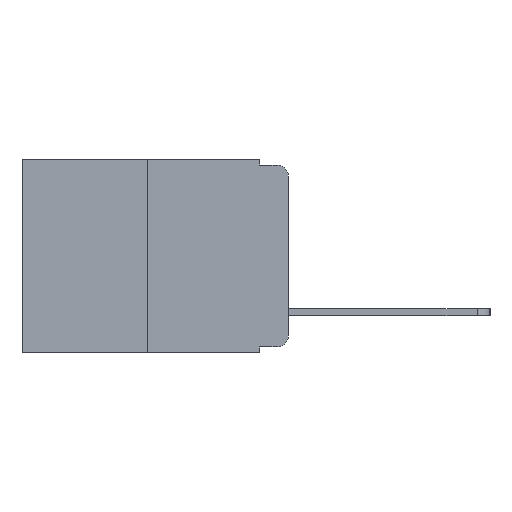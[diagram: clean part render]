
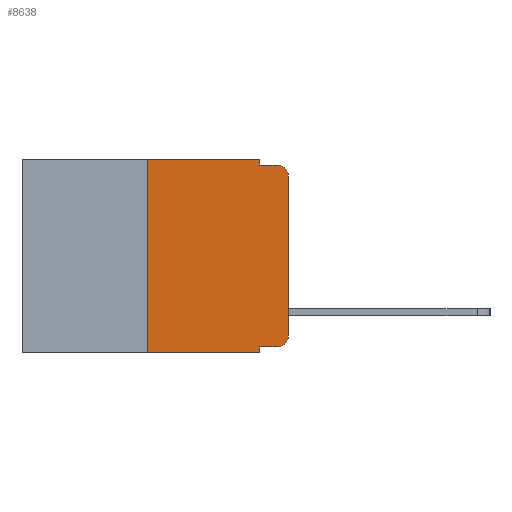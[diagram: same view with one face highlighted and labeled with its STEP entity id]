
A CAD part, left-side view. The second image highlights one B-rep face of the part: STEP entity #8638.
In plain terms, the highlighted planar face has unit normal (-1, 0, 0).
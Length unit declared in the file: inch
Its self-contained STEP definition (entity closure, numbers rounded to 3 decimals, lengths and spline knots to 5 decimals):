
#238 = ORIENTED_EDGE ( 'NONE', *, *, #7026, .T. ) ;
#520 = CARTESIAN_POINT ( 'NONE',  ( 0., 0.02, -0.01 ) ) ;
#692 = VERTEX_POINT ( 'NONE', #14526 ) ;
#790 = AXIS2_PLACEMENT_3D ( 'NONE', #9819, #8954, #10452 ) ;
#845 = CARTESIAN_POINT ( 'NONE',  ( 0., 0.051, -0.343 ) ) ;
#1136 = EDGE_CURVE ( 'NONE', #4900, #7014, #1927, .T. ) ;
#1307 = EDGE_CURVE ( 'NONE', #6296, #9072, #5280, .T. ) ;
#1420 = VERTEX_POINT ( 'NONE', #9366 ) ;
#1461 = VECTOR ( 'NONE', #11084, 39.37008 ) ;
#1786 = VERTEX_POINT ( 'NONE', #845 ) ;
#1927 = LINE ( 'NONE', #8171, #4402 ) ;
#2137 = DIRECTION ( 'NONE',  ( 0., 0., 1. ) ) ;
#2161 = EDGE_CURVE ( 'NONE', #1420, #6296, #7194, .T. ) ;
#2955 = EDGE_CURVE ( 'NONE', #1420, #1786, #13130, .T. ) ;
#3192 = VECTOR ( 'NONE', #13344, 39.37008 ) ;
#3286 = EDGE_LOOP ( 'NONE', ( #238, #3532, #9862, #3923, #10218, #7521, #10550, #4678, #7887, #10880 ) ) ;
#3414 = LINE ( 'NONE', #9518, #6639 ) ;
#3532 = ORIENTED_EDGE ( 'NONE', *, *, #6193, .T. ) ;
#3570 = DIRECTION ( 'NONE',  ( 0., 0., 1. ) ) ;
#3774 = EDGE_CURVE ( 'NONE', #8325, #4900, #13782, .T. ) ;
#3923 = ORIENTED_EDGE ( 'NONE', *, *, #4597, .F. ) ;
#3957 = VERTEX_POINT ( 'NONE', #3966 ) ;
#3966 = CARTESIAN_POINT ( 'NONE',  ( 0., 0.051, -0.01 ) ) ;
#4151 = VERTEX_POINT ( 'NONE', #520 ) ;
#4402 = VECTOR ( 'NONE', #12120, 39.37008 ) ;
#4597 = EDGE_CURVE ( 'NONE', #7014, #3957, #11604, .T. ) ;
#4678 = ORIENTED_EDGE ( 'NONE', *, *, #2955, .F. ) ;
#4755 = DIRECTION ( 'NONE',  ( 1., 0., 0. ) ) ;
#4900 = VERTEX_POINT ( 'NONE', #9797 ) ;
#4984 = CARTESIAN_POINT ( 'NONE',  ( 0., 0.051, 0. ) ) ;
#5280 = CIRCLE ( 'NONE', #7171, 0.02 ) ;
#5340 = EDGE_CURVE ( 'NONE', #3957, #4151, #7539, .T. ) ;
#5543 = VECTOR ( 'NONE', #12682, 39.37008 ) ;
#5758 = DIRECTION ( 'NONE',  ( 0., -1., 0. ) ) ;
#5847 = CARTESIAN_POINT ( 'NONE',  ( 0., 0.473, -0.343 ) ) ;
#5902 = CARTESIAN_POINT ( 'NONE',  ( 0., 0.473, 0. ) ) ;
#6043 = CARTESIAN_POINT ( 'NONE',  ( 0., 0.02, -0.333 ) ) ;
#6193 = EDGE_CURVE ( 'NONE', #692, #4151, #8879, .T. ) ;
#6296 = VERTEX_POINT ( 'NONE', #6043 ) ;
#6639 = VECTOR ( 'NONE', #3570, 39.37008 ) ;
#7014 = VERTEX_POINT ( 'NONE', #7164 ) ;
#7026 = EDGE_CURVE ( 'NONE', #9072, #692, #3414, .T. ) ;
#7164 = CARTESIAN_POINT ( 'NONE',  ( 0., 0.051, 0. ) ) ;
#7171 = AXIS2_PLACEMENT_3D ( 'NONE', #14013, #14075, #14631 ) ;
#7194 = LINE ( 'NONE', #11792, #12797 ) ;
#7521 = ORIENTED_EDGE ( 'NONE', *, *, #3774, .F. ) ;
#7539 = LINE ( 'NONE', #13043, #1461 ) ;
#7887 = ORIENTED_EDGE ( 'NONE', *, *, #2161, .T. ) ;
#7933 = VECTOR ( 'NONE', #2137, 39.37008 ) ;
#8015 = FACE_OUTER_BOUND ( 'NONE', #3286, .T. ) ;
#8171 = CARTESIAN_POINT ( 'NONE',  ( 0., 0.473, 0. ) ) ;
#8325 = VERTEX_POINT ( 'NONE', #13309 ) ;
#8364 = DIRECTION ( 'NONE',  ( 0., 0., -1. ) ) ;
#8397 = LINE ( 'NONE', #5847, #5543 ) ;
#8638 = ADVANCED_FACE ( 'NONE', ( #8015 ), #9487, .F. ) ;
#8879 = CIRCLE ( 'NONE', #790, 0.02 ) ;
#8954 = DIRECTION ( 'NONE',  ( -1., 0., 0. ) ) ;
#9072 = VERTEX_POINT ( 'NONE', #13862 ) ;
#9366 = CARTESIAN_POINT ( 'NONE',  ( 0., 0.051, -0.333 ) ) ;
#9487 = PLANE ( 'NONE',  #10616 ) ;
#9518 = CARTESIAN_POINT ( 'NONE',  ( 0., 0., 0. ) ) ;
#9797 = CARTESIAN_POINT ( 'NONE',  ( 0., 0.25, 0. ) ) ;
#9819 = CARTESIAN_POINT ( 'NONE',  ( 0., 0.02, -0.03 ) ) ;
#9862 = ORIENTED_EDGE ( 'NONE', *, *, #5340, .F. ) ;
#10218 = ORIENTED_EDGE ( 'NONE', *, *, #1136, .F. ) ;
#10452 = DIRECTION ( 'NONE',  ( 0., 0., -1. ) ) ;
#10550 = ORIENTED_EDGE ( 'NONE', *, *, #14178, .T. ) ;
#10616 = AXIS2_PLACEMENT_3D ( 'NONE', #5902, #4755, #12763 ) ;
#10880 = ORIENTED_EDGE ( 'NONE', *, *, #1307, .T. ) ;
#10910 = CARTESIAN_POINT ( 'NONE',  ( 0., 0.25, 0. ) ) ;
#11084 = DIRECTION ( 'NONE',  ( 0., -1., 0. ) ) ;
#11604 = LINE ( 'NONE', #13112, #14104 ) ;
#11792 = CARTESIAN_POINT ( 'NONE',  ( 0., 0.051, -0.333 ) ) ;
#12120 = DIRECTION ( 'NONE',  ( 0., -1., 0. ) ) ;
#12682 = DIRECTION ( 'NONE',  ( 0., -1., 0. ) ) ;
#12763 = DIRECTION ( 'NONE',  ( 0., 0., -1. ) ) ;
#12797 = VECTOR ( 'NONE', #5758, 39.37008 ) ;
#13043 = CARTESIAN_POINT ( 'NONE',  ( 0., 0.051, -0.01 ) ) ;
#13112 = CARTESIAN_POINT ( 'NONE',  ( 0., 0.051, 0. ) ) ;
#13130 = LINE ( 'NONE', #4984, #3192 ) ;
#13309 = CARTESIAN_POINT ( 'NONE',  ( 0., 0.25, -0.343 ) ) ;
#13344 = DIRECTION ( 'NONE',  ( 0., 0., -1. ) ) ;
#13782 = LINE ( 'NONE', #10910, #7933 ) ;
#13862 = CARTESIAN_POINT ( 'NONE',  ( 0., 0., -0.313 ) ) ;
#14013 = CARTESIAN_POINT ( 'NONE',  ( 0., 0.02, -0.313 ) ) ;
#14075 = DIRECTION ( 'NONE',  ( -1., 0., 0. ) ) ;
#14104 = VECTOR ( 'NONE', #8364, 39.37008 ) ;
#14178 = EDGE_CURVE ( 'NONE', #8325, #1786, #8397, .T. ) ;
#14526 = CARTESIAN_POINT ( 'NONE',  ( 0., 0., -0.03 ) ) ;
#14631 = DIRECTION ( 'NONE',  ( 0., 0., -1. ) ) ;
